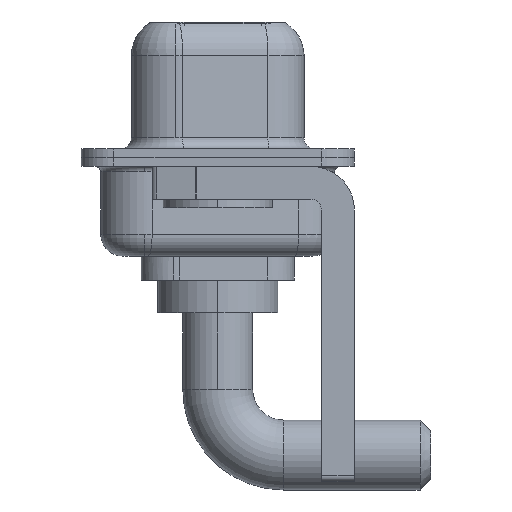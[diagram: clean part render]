
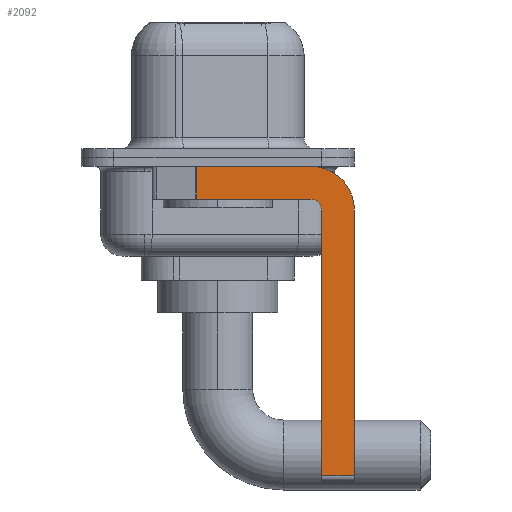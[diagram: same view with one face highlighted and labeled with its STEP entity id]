
A CAD part, left-side view. The second image highlights one B-rep face of the part: STEP entity #2092.
In plain terms, the highlighted planar face has unit normal (-1, 0, 0).
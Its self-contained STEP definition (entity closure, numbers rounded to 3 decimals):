
#111 = ORIENTED_EDGE ( 'NONE', *, *, #5111, .F. ) ;
#154 = VERTEX_POINT ( 'NONE', #5583 ) ;
#168 = CIRCLE ( 'NONE', #6825, 0.5 ) ;
#613 = DIRECTION ( 'NONE',  ( 0., -1., 0. ) ) ;
#751 = PLANE ( 'NONE',  #6447 ) ;
#821 = EDGE_CURVE ( 'NONE', #8735, #10574, #4161, .T. ) ;
#957 = VERTEX_POINT ( 'NONE', #1389 ) ;
#1389 = CARTESIAN_POINT ( 'NONE',  ( -2.9, 0.978, -0.4 ) ) ;
#1477 = CARTESIAN_POINT ( 'NONE',  ( -2.9, -4.25, -14.55 ) ) ;
#1552 = CIRCLE ( 'NONE', #4900, 2. ) ;
#1737 = DIRECTION ( 'NONE',  ( 0., 0., -1. ) ) ;
#1902 = CARTESIAN_POINT ( 'NONE',  ( -2.9, -4.25, -2.4 ) ) ;
#2024 = DIRECTION ( 'NONE',  ( 1., 0., 0. ) ) ;
#2092 = ADVANCED_FACE ( 'NONE', ( #12711 ), #751, .F. ) ;
#2132 = ORIENTED_EDGE ( 'NONE', *, *, #3267, .F. ) ;
#2347 = EDGE_CURVE ( 'NONE', #3828, #154, #4580, .T. ) ;
#2430 = LINE ( 'NONE', #4388, #6684 ) ;
#2449 = LINE ( 'NONE', #1477, #10723 ) ;
#2488 = DIRECTION ( 'NONE',  ( 0., 1., 0. ) ) ;
#3122 = DIRECTION ( 'NONE',  ( 0., 0., -1. ) ) ;
#3267 = EDGE_CURVE ( 'NONE', #957, #11355, #10535, .T. ) ;
#3654 = VERTEX_POINT ( 'NONE', #7336 ) ;
#3828 = VERTEX_POINT ( 'NONE', #6608 ) ;
#3911 = CARTESIAN_POINT ( 'NONE',  ( -2.9, -4.25, -2.4 ) ) ;
#4161 = LINE ( 'NONE', #9256, #10796 ) ;
#4388 = CARTESIAN_POINT ( 'NONE',  ( -2.9, -4.75, -14.8 ) ) ;
#4462 = CARTESIAN_POINT ( 'NONE',  ( -2.9, -4.75, -14.55 ) ) ;
#4580 = LINE ( 'NONE', #9672, #6655 ) ;
#4900 = AXIS2_PLACEMENT_3D ( 'NONE', #1902, #2024, #5031 ) ;
#5005 = ORIENTED_EDGE ( 'NONE', *, *, #11936, .T. ) ;
#5031 = DIRECTION ( 'NONE',  ( 0., 0., -1. ) ) ;
#5111 = EDGE_CURVE ( 'NONE', #8997, #3654, #2430, .T. ) ;
#5269 = ORIENTED_EDGE ( 'NONE', *, *, #7934, .T. ) ;
#5583 = CARTESIAN_POINT ( 'NONE',  ( -2.9, 0.978, -1.9 ) ) ;
#5652 = EDGE_CURVE ( 'NONE', #3654, #3828, #168, .T. ) ;
#5978 = ORIENTED_EDGE ( 'NONE', *, *, #821, .F. ) ;
#6257 = VECTOR ( 'NONE', #613, 1000. ) ;
#6447 = AXIS2_PLACEMENT_3D ( 'NONE', #6831, #10807, #1737 ) ;
#6511 = DIRECTION ( 'NONE',  ( 0., -1., 0. ) ) ;
#6608 = CARTESIAN_POINT ( 'NONE',  ( -2.9, -4.25, -1.9 ) ) ;
#6655 = VECTOR ( 'NONE', #2488, 1000. ) ;
#6684 = VECTOR ( 'NONE', #8383, 1000. ) ;
#6695 = CARTESIAN_POINT ( 'NONE',  ( -2.9, 3., -0.4 ) ) ;
#6825 = AXIS2_PLACEMENT_3D ( 'NONE', #3911, #12942, #9981 ) ;
#6831 = CARTESIAN_POINT ( 'NONE',  ( -2.9, -4.25, -2.4 ) ) ;
#6842 = ORIENTED_EDGE ( 'NONE', *, *, #7234, .F. ) ;
#7044 = LINE ( 'NONE', #11017, #11511 ) ;
#7234 = EDGE_CURVE ( 'NONE', #11355, #8735, #1552, .T. ) ;
#7280 = CARTESIAN_POINT ( 'NONE',  ( -2.9, -6.25, -2.4 ) ) ;
#7336 = CARTESIAN_POINT ( 'NONE',  ( -2.9, -4.75, -2.4 ) ) ;
#7934 = EDGE_CURVE ( 'NONE', #8997, #10574, #2449, .T. ) ;
#8383 = DIRECTION ( 'NONE',  ( 0., 0., 1. ) ) ;
#8702 = CARTESIAN_POINT ( 'NONE',  ( -2.9, -6.25, -14.55 ) ) ;
#8735 = VERTEX_POINT ( 'NONE', #7280 ) ;
#8997 = VERTEX_POINT ( 'NONE', #4462 ) ;
#9256 = CARTESIAN_POINT ( 'NONE',  ( -2.9, -6.25, -2.4 ) ) ;
#9393 = ORIENTED_EDGE ( 'NONE', *, *, #2347, .F. ) ;
#9672 = CARTESIAN_POINT ( 'NONE',  ( -2.9, -4.25, -1.9 ) ) ;
#9734 = ORIENTED_EDGE ( 'NONE', *, *, #5652, .F. ) ;
#9981 = DIRECTION ( 'NONE',  ( 0., 0., 1. ) ) ;
#10357 = DIRECTION ( 'NONE',  ( 0., 0., -1. ) ) ;
#10535 = LINE ( 'NONE', #6695, #6257 ) ;
#10574 = VERTEX_POINT ( 'NONE', #8702 ) ;
#10723 = VECTOR ( 'NONE', #6511, 1000. ) ;
#10796 = VECTOR ( 'NONE', #3122, 1000. ) ;
#10807 = DIRECTION ( 'NONE',  ( 1., 0., 0. ) ) ;
#11017 = CARTESIAN_POINT ( 'NONE',  ( -2.9, 0.978, -1.9 ) ) ;
#11355 = VERTEX_POINT ( 'NONE', #11961 ) ;
#11511 = VECTOR ( 'NONE', #10357, 1000. ) ;
#11936 = EDGE_CURVE ( 'NONE', #957, #154, #7044, .T. ) ;
#11961 = CARTESIAN_POINT ( 'NONE',  ( -2.9, -4.25, -0.4 ) ) ;
#11967 = EDGE_LOOP ( 'NONE', ( #2132, #5005, #9393, #9734, #111, #5269, #5978, #6842 ) ) ;
#12711 = FACE_OUTER_BOUND ( 'NONE', #11967, .T. ) ;
#12942 = DIRECTION ( 'NONE',  ( -1., 0., 0. ) ) ;
